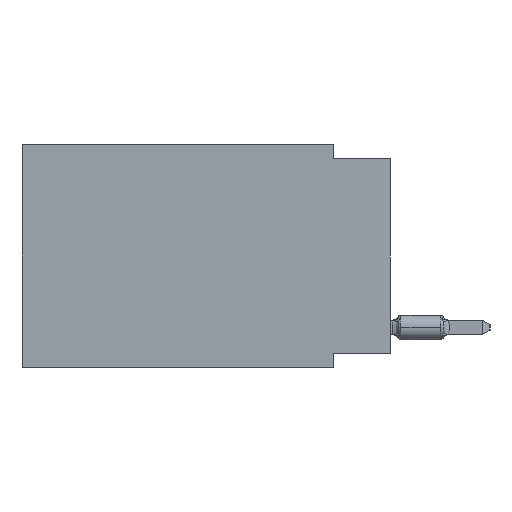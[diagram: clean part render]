
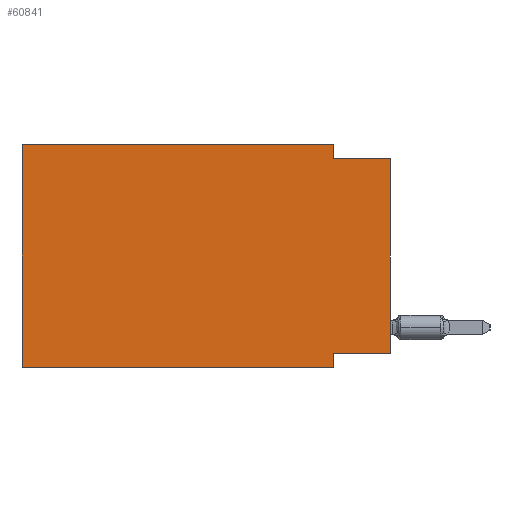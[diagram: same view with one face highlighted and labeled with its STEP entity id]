
A CAD part, left-side view. The second image highlights one B-rep face of the part: STEP entity #60841.
In plain terms, the highlighted planar face has unit normal (-1, 0, 0).
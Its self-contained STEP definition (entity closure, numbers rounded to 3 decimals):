
#827 = ORIENTED_EDGE ( 'NONE', *, *, #27768, .F. ) ;
#1665 = VERTEX_POINT ( 'NONE', #9260 ) ;
#1925 = LINE ( 'NONE', #60148, #13654 ) ;
#2810 = CARTESIAN_POINT ( 'NONE',  ( 0., 2.54, -0.635 ) ) ;
#2843 = VECTOR ( 'NONE', #3018, 1000. ) ;
#3017 = ORIENTED_EDGE ( 'NONE', *, *, #59718, .F. ) ;
#3018 = DIRECTION ( 'NONE',  ( 0., 0., -1. ) ) ;
#3562 = VERTEX_POINT ( 'NONE', #49455 ) ;
#3816 = VERTEX_POINT ( 'NONE', #35486 ) ;
#5589 = EDGE_CURVE ( 'NONE', #3562, #24044, #41644, .T. ) ;
#5996 = VERTEX_POINT ( 'NONE', #60386 ) ;
#6319 = CARTESIAN_POINT ( 'NONE',  ( 0., 2.54, -9.271 ) ) ;
#9260 = CARTESIAN_POINT ( 'NONE',  ( 0., 2.54, 0. ) ) ;
#13424 = DIRECTION ( 'NONE',  ( 1., 0., 0. ) ) ;
#13654 = VECTOR ( 'NONE', #55265, 1000. ) ;
#13978 = CARTESIAN_POINT ( 'NONE',  ( 0., 16.383, 0. ) ) ;
#15181 = DIRECTION ( 'NONE',  ( 0., 0., 1. ) ) ;
#15240 = AXIS2_PLACEMENT_3D ( 'NONE', #35710, #13424, #55605 ) ;
#18761 = VECTOR ( 'NONE', #32547, 1000. ) ;
#20909 = VECTOR ( 'NONE', #35551, 1000. ) ;
#23929 = DIRECTION ( 'NONE',  ( 0., 0., 1. ) ) ;
#24044 = VERTEX_POINT ( 'NONE', #57636 ) ;
#24225 = FACE_OUTER_BOUND ( 'NONE', #67058, .T. ) ;
#24620 = LINE ( 'NONE', #40965, #2843 ) ;
#24903 = ORIENTED_EDGE ( 'NONE', *, *, #60606, .T. ) ;
#27768 = EDGE_CURVE ( 'NONE', #1665, #40869, #55909, .T. ) ;
#28700 = DIRECTION ( 'NONE',  ( 0., 0., -1. ) ) ;
#29091 = PLANE ( 'NONE',  #15240 ) ;
#29400 = CARTESIAN_POINT ( 'NONE',  ( 0., 2.54, 0. ) ) ;
#29506 = EDGE_CURVE ( 'NONE', #3562, #59374, #36940, .T. ) ;
#30870 = CARTESIAN_POINT ( 'NONE',  ( 0., 0., 0. ) ) ;
#32547 = DIRECTION ( 'NONE',  ( 0., -1., 0. ) ) ;
#33083 = DIRECTION ( 'NONE',  ( 0., 1., 0. ) ) ;
#35486 = CARTESIAN_POINT ( 'NONE',  ( 0., 0., -0.635 ) ) ;
#35551 = DIRECTION ( 'NONE',  ( 0., -1., 0. ) ) ;
#35710 = CARTESIAN_POINT ( 'NONE',  ( 0., 16.383, 0. ) ) ;
#36756 = CARTESIAN_POINT ( 'NONE',  ( 0., 16.383, -9.906 ) ) ;
#36940 = LINE ( 'NONE', #56680, #38825 ) ;
#37907 = VERTEX_POINT ( 'NONE', #6319 ) ;
#38825 = VECTOR ( 'NONE', #23929, 1000. ) ;
#40429 = CARTESIAN_POINT ( 'NONE',  ( 0., 0., -0.635 ) ) ;
#40869 = VERTEX_POINT ( 'NONE', #2810 ) ;
#40965 = CARTESIAN_POINT ( 'NONE',  ( 0., 2.54, -9.906 ) ) ;
#40981 = EDGE_CURVE ( 'NONE', #40869, #3816, #46010, .T. ) ;
#41644 = LINE ( 'NONE', #36756, #18761 ) ;
#42854 = LINE ( 'NONE', #58902, #58010 ) ;
#46010 = LINE ( 'NONE', #40429, #20909 ) ;
#46335 = EDGE_CURVE ( 'NONE', #59374, #1665, #1925, .T. ) ;
#46887 = LINE ( 'NONE', #30870, #67499 ) ;
#47717 = VECTOR ( 'NONE', #28700, 1000. ) ;
#49254 = ORIENTED_EDGE ( 'NONE', *, *, #46335, .F. ) ;
#49455 = CARTESIAN_POINT ( 'NONE',  ( 0., 16.383, -9.906 ) ) ;
#55265 = DIRECTION ( 'NONE',  ( 0., -1., 0. ) ) ;
#55605 = DIRECTION ( 'NONE',  ( 0., 0., -1. ) ) ;
#55909 = LINE ( 'NONE', #29400, #47717 ) ;
#56680 = CARTESIAN_POINT ( 'NONE',  ( 0., 16.383, 0. ) ) ;
#56825 = EDGE_CURVE ( 'NONE', #5996, #37907, #42854, .T. ) ;
#57636 = CARTESIAN_POINT ( 'NONE',  ( 0., 2.54, -9.906 ) ) ;
#58010 = VECTOR ( 'NONE', #33083, 1000. ) ;
#58902 = CARTESIAN_POINT ( 'NONE',  ( 0., 0., -9.271 ) ) ;
#59374 = VERTEX_POINT ( 'NONE', #13978 ) ;
#59718 = EDGE_CURVE ( 'NONE', #37907, #24044, #24620, .T. ) ;
#60148 = CARTESIAN_POINT ( 'NONE',  ( 0., 16.383, 0. ) ) ;
#60386 = CARTESIAN_POINT ( 'NONE',  ( 0., 0., -9.271 ) ) ;
#60553 = ORIENTED_EDGE ( 'NONE', *, *, #5589, .T. ) ;
#60606 = EDGE_CURVE ( 'NONE', #5996, #3816, #46887, .T. ) ;
#60841 = ADVANCED_FACE ( 'NONE', ( #24225 ), #29091, .F. ) ;
#64735 = ORIENTED_EDGE ( 'NONE', *, *, #56825, .F. ) ;
#65405 = ORIENTED_EDGE ( 'NONE', *, *, #29506, .F. ) ;
#65798 = ORIENTED_EDGE ( 'NONE', *, *, #40981, .F. ) ;
#67058 = EDGE_LOOP ( 'NONE', ( #24903, #65798, #827, #49254, #65405, #60553, #3017, #64735 ) ) ;
#67499 = VECTOR ( 'NONE', #15181, 1000. ) ;
